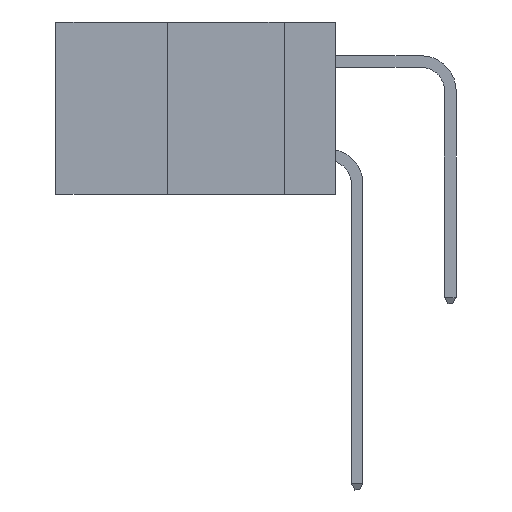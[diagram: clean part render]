
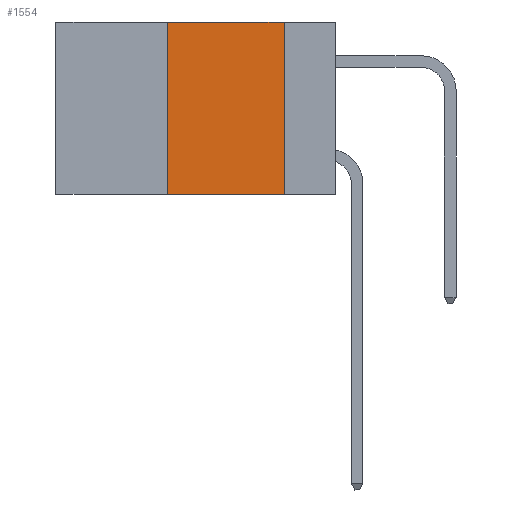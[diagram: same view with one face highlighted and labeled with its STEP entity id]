
A CAD part, left-side view. The second image highlights one B-rep face of the part: STEP entity #1554.
In plain terms, the highlighted planar face has unit normal (-1, 0, 0).
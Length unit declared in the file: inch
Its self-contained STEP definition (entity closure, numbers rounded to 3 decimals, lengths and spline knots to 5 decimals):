
#51 = CARTESIAN_POINT ( 'NONE',  ( 0., 0.36, 0. ) ) ;
#949 = CARTESIAN_POINT ( 'NONE',  ( 0., 0.6, -0.37 ) ) ;
#1554 = ADVANCED_FACE ( 'NONE', ( #3199 ), #15309, .F. ) ;
#2915 = VERTEX_POINT ( 'NONE', #13101 ) ;
#3199 = FACE_OUTER_BOUND ( 'NONE', #16691, .T. ) ;
#3241 = DIRECTION ( 'NONE',  ( 1., 0., 0. ) ) ;
#3537 = VERTEX_POINT ( 'NONE', #51 ) ;
#4367 = CARTESIAN_POINT ( 'NONE',  ( 0., 0.11, 0. ) ) ;
#4429 = AXIS2_PLACEMENT_3D ( 'NONE', #11968, #3241, #16887 ) ;
#4477 = VECTOR ( 'NONE', #18641, 39.37008 ) ;
#7148 = CARTESIAN_POINT ( 'NONE',  ( 0., 0.36, 0. ) ) ;
#9420 = VECTOR ( 'NONE', #14044, 39.37008 ) ;
#9518 = CARTESIAN_POINT ( 'NONE',  ( 0., 0.11, 0. ) ) ;
#10222 = CARTESIAN_POINT ( 'NONE',  ( 0., 0.6, 0. ) ) ;
#10927 = ORIENTED_EDGE ( 'NONE', *, *, #21254, .F. ) ;
#11008 = VERTEX_POINT ( 'NONE', #12000 ) ;
#11355 = EDGE_CURVE ( 'NONE', #22354, #11008, #20685, .T. ) ;
#11681 = VECTOR ( 'NONE', #17952, 39.37008 ) ;
#11968 = CARTESIAN_POINT ( 'NONE',  ( 0., 0.6, 0. ) ) ;
#12000 = CARTESIAN_POINT ( 'NONE',  ( 0., 0.11, -0.37 ) ) ;
#13048 = ORIENTED_EDGE ( 'NONE', *, *, #22240, .T. ) ;
#13101 = CARTESIAN_POINT ( 'NONE',  ( 0., 0.36, -0.37 ) ) ;
#13594 = LINE ( 'NONE', #949, #17500 ) ;
#14044 = DIRECTION ( 'NONE',  ( 0., 0., 1. ) ) ;
#14912 = DIRECTION ( 'NONE',  ( 0., -1., 0. ) ) ;
#15309 = PLANE ( 'NONE',  #4429 ) ;
#16690 = ORIENTED_EDGE ( 'NONE', *, *, #20093, .F. ) ;
#16691 = EDGE_LOOP ( 'NONE', ( #21253, #10927, #16690, #13048 ) ) ;
#16887 = DIRECTION ( 'NONE',  ( 0., 0., -1. ) ) ;
#17500 = VECTOR ( 'NONE', #14912, 39.37008 ) ;
#17893 = LINE ( 'NONE', #7148, #9420 ) ;
#17952 = DIRECTION ( 'NONE',  ( 0., 0., -1. ) ) ;
#18641 = DIRECTION ( 'NONE',  ( 0., -1., 0. ) ) ;
#20093 = EDGE_CURVE ( 'NONE', #2915, #3537, #17893, .T. ) ;
#20685 = LINE ( 'NONE', #9518, #11681 ) ;
#21253 = ORIENTED_EDGE ( 'NONE', *, *, #11355, .F. ) ;
#21254 = EDGE_CURVE ( 'NONE', #3537, #22354, #22097, .T. ) ;
#22097 = LINE ( 'NONE', #10222, #4477 ) ;
#22240 = EDGE_CURVE ( 'NONE', #2915, #11008, #13594, .T. ) ;
#22354 = VERTEX_POINT ( 'NONE', #4367 ) ;
